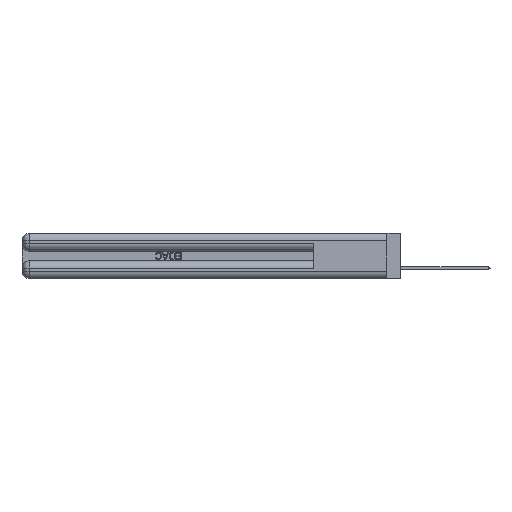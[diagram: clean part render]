
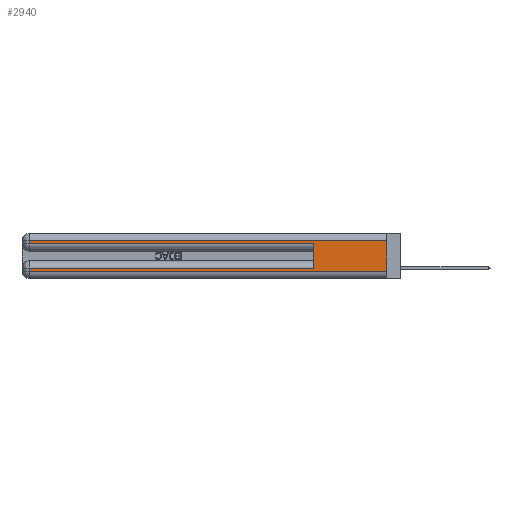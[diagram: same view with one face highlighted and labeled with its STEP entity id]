
A CAD part, left-side view. The second image highlights one B-rep face of the part: STEP entity #2940.
In plain terms, the highlighted planar face has unit normal (-1, 0, 0).
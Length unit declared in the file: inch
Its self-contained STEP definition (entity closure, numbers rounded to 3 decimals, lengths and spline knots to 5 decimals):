
#1343 = CARTESIAN_POINT ( 'NONE',  ( 0., 2.94, 0.31 ) ) ;
#1569 = VERTEX_POINT ( 'NONE', #3169 ) ;
#2445 = CARTESIAN_POINT ( 'NONE',  ( 0., 2.94, 0.285 ) ) ;
#2886 = ORIENTED_EDGE ( 'NONE', *, *, #27795, .F. ) ;
#2940 = ADVANCED_FACE ( 'NONE', ( #6277 ), #44078, .F. ) ;
#3169 = CARTESIAN_POINT ( 'NONE',  ( 0., 0., 0.31 ) ) ;
#3725 = LINE ( 'NONE', #20856, #5068 ) ;
#5068 = VECTOR ( 'NONE', #29141, 39.37008 ) ;
#6277 = FACE_OUTER_BOUND ( 'NONE', #28843, .T. ) ;
#7170 = VECTOR ( 'NONE', #9423, 39.37008 ) ;
#7181 = ORIENTED_EDGE ( 'NONE', *, *, #28961, .T. ) ;
#8423 = VECTOR ( 'NONE', #19580, 39.37008 ) ;
#9423 = DIRECTION ( 'NONE',  ( 0., 0., -1. ) ) ;
#9588 = VERTEX_POINT ( 'NONE', #37384 ) ;
#10886 = CARTESIAN_POINT ( 'NONE',  ( 0., 2.94, 0.06 ) ) ;
#10984 = LINE ( 'NONE', #45876, #39721 ) ;
#12245 = DIRECTION ( 'NONE',  ( 0., 0., -1. ) ) ;
#13863 = EDGE_CURVE ( 'NONE', #47667, #9588, #3725, .T. ) ;
#13870 = ORIENTED_EDGE ( 'NONE', *, *, #14234, .T. ) ;
#14234 = EDGE_CURVE ( 'NONE', #1569, #29986, #53080, .T. ) ;
#14893 = DIRECTION ( 'NONE',  ( 1., 0., 0. ) ) ;
#15035 = DIRECTION ( 'NONE',  ( 0., 1., 0. ) ) ;
#15713 = EDGE_CURVE ( 'NONE', #38764, #26753, #49863, .T. ) ;
#16461 = EDGE_CURVE ( 'NONE', #29986, #41778, #10984, .T. ) ;
#19580 = DIRECTION ( 'NONE',  ( 0., 0., 1. ) ) ;
#20856 = CARTESIAN_POINT ( 'NONE',  ( 0., 0., 0.06 ) ) ;
#24328 = LINE ( 'NONE', #37081, #42408 ) ;
#24821 = DIRECTION ( 'NONE',  ( 0., 1., 0. ) ) ;
#25202 = LINE ( 'NONE', #31301, #7170 ) ;
#26596 = CARTESIAN_POINT ( 'NONE',  ( 0., 0.6, 0.285 ) ) ;
#26712 = CARTESIAN_POINT ( 'NONE',  ( 0., 0.6, 0.085 ) ) ;
#26753 = VERTEX_POINT ( 'NONE', #30568 ) ;
#27790 = VECTOR ( 'NONE', #24821, 39.37008 ) ;
#27795 = EDGE_CURVE ( 'NONE', #38764, #50511, #45250, .T. ) ;
#27999 = AXIS2_PLACEMENT_3D ( 'NONE', #36199, #14893, #31565 ) ;
#28843 = EDGE_LOOP ( 'NONE', ( #36535, #13870, #37787, #7181, #2886, #51988, #49260, #39800 ) ) ;
#28961 = EDGE_CURVE ( 'NONE', #41778, #50511, #24328, .T. ) ;
#29141 = DIRECTION ( 'NONE',  ( 0., -1., 0. ) ) ;
#29986 = VERTEX_POINT ( 'NONE', #1343 ) ;
#30405 = VECTOR ( 'NONE', #15035, 39.37008 ) ;
#30568 = CARTESIAN_POINT ( 'NONE',  ( 0., 2.94, 0.085 ) ) ;
#31301 = CARTESIAN_POINT ( 'NONE',  ( 0., 2.94, 0.37 ) ) ;
#31565 = DIRECTION ( 'NONE',  ( 0., 0., -1. ) ) ;
#33048 = CARTESIAN_POINT ( 'NONE',  ( 0., 0.6, 0.145 ) ) ;
#36199 = CARTESIAN_POINT ( 'NONE',  ( 0., 0., 0.37 ) ) ;
#36535 = ORIENTED_EDGE ( 'NONE', *, *, #36944, .F. ) ;
#36944 = EDGE_CURVE ( 'NONE', #1569, #9588, #54927, .T. ) ;
#37081 = CARTESIAN_POINT ( 'NONE',  ( 0., 0., 0.285 ) ) ;
#37384 = CARTESIAN_POINT ( 'NONE',  ( 0., 0., 0.06 ) ) ;
#37787 = ORIENTED_EDGE ( 'NONE', *, *, #16461, .T. ) ;
#38764 = VERTEX_POINT ( 'NONE', #26712 ) ;
#39721 = VECTOR ( 'NONE', #50164, 39.37008 ) ;
#39800 = ORIENTED_EDGE ( 'NONE', *, *, #13863, .T. ) ;
#41601 = DIRECTION ( 'NONE',  ( 0., -1., 0. ) ) ;
#41622 = CARTESIAN_POINT ( 'NONE',  ( 0., 0., 0.37 ) ) ;
#41778 = VERTEX_POINT ( 'NONE', #2445 ) ;
#42022 = CARTESIAN_POINT ( 'NONE',  ( 0., 0., 0.085 ) ) ;
#42408 = VECTOR ( 'NONE', #41601, 39.37008 ) ;
#44078 = PLANE ( 'NONE',  #27999 ) ;
#45136 = CARTESIAN_POINT ( 'NONE',  ( 0., 0., 0.31 ) ) ;
#45250 = LINE ( 'NONE', #33048, #8423 ) ;
#45876 = CARTESIAN_POINT ( 'NONE',  ( 0., 2.94, 0.37 ) ) ;
#47667 = VERTEX_POINT ( 'NONE', #10886 ) ;
#48254 = VECTOR ( 'NONE', #12245, 39.37008 ) ;
#49233 = EDGE_CURVE ( 'NONE', #26753, #47667, #25202, .T. ) ;
#49260 = ORIENTED_EDGE ( 'NONE', *, *, #49233, .T. ) ;
#49863 = LINE ( 'NONE', #42022, #27790 ) ;
#50164 = DIRECTION ( 'NONE',  ( 0., 0., -1. ) ) ;
#50511 = VERTEX_POINT ( 'NONE', #26596 ) ;
#51988 = ORIENTED_EDGE ( 'NONE', *, *, #15713, .T. ) ;
#53080 = LINE ( 'NONE', #45136, #30405 ) ;
#54927 = LINE ( 'NONE', #41622, #48254 ) ;
